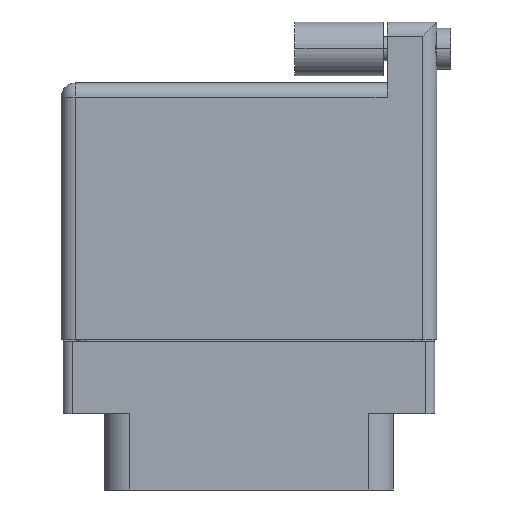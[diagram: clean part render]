
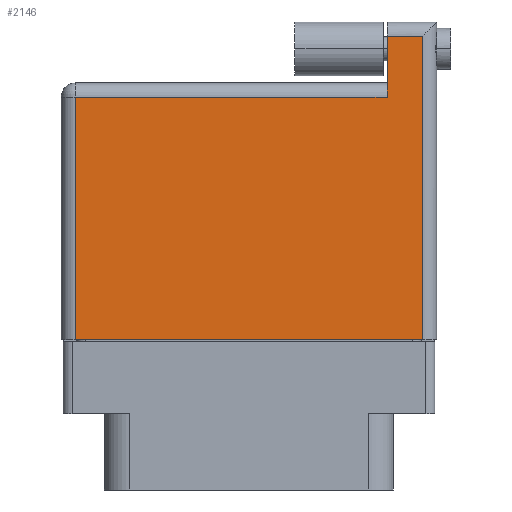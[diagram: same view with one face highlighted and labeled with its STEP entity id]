
A CAD part, front view. The second image highlights one B-rep face of the part: STEP entity #2146.
In plain terms, the highlighted face is planar.
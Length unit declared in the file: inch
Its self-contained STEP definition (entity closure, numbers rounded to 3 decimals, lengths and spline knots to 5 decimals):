
#5 = EDGE_CURVE ( 'NONE', #26352, #6778, #14544, .T. ) ;
#2075 = AXIS2_PLACEMENT_3D ( 'NONE', #9101, #6784, #22873 ) ;
#2146 = ADVANCED_FACE ( 'NONE', ( #16051 ), #13891, .F. ) ;
#3312 = VERTEX_POINT ( 'NONE', #17514 ) ;
#4129 = CARTESIAN_POINT ( 'NONE',  ( -0.6625, 0.97, 0.3575 ) ) ;
#5435 = CARTESIAN_POINT ( 'NONE',  ( 0.4875, 1.02, 0.3575 ) ) ;
#6078 = CARTESIAN_POINT ( 'NONE',  ( -0.6125, -0.1, 0.3575 ) ) ;
#6567 = CARTESIAN_POINT ( 'NONE',  ( 0.4875, 0.97, 0.3575 ) ) ;
#6591 = LINE ( 'NONE', #4129, #15078 ) ;
#6778 = VERTEX_POINT ( 'NONE', #12394 ) ;
#6784 = DIRECTION ( 'NONE',  ( 0., 0., -1. ) ) ;
#7570 = EDGE_CURVE ( 'NONE', #29473, #29462, #14481, .T. ) ;
#8029 = EDGE_CURVE ( 'NONE', #26629, #29473, #13776, .T. ) ;
#8240 = VECTOR ( 'NONE', #25083, 39.37008 ) ;
#9101 = CARTESIAN_POINT ( 'NONE',  ( -0.6625, 0.806, 0.3575 ) ) ;
#9293 = VECTOR ( 'NONE', #26597, 39.37008 ) ;
#10101 = ORIENTED_EDGE ( 'NONE', *, *, #7570, .T. ) ;
#10362 = LINE ( 'NONE', #17004, #9293 ) ;
#11129 = ORIENTED_EDGE ( 'NONE', *, *, #21129, .T. ) ;
#12394 = CARTESIAN_POINT ( 'NONE',  ( 0.4875, 0.756, 0.3575 ) ) ;
#12858 = ORIENTED_EDGE ( 'NONE', *, *, #5, .T. ) ;
#13776 = LINE ( 'NONE', #23210, #20908 ) ;
#13891 = PLANE ( 'NONE',  #2075 ) ;
#14118 = CARTESIAN_POINT ( 'NONE',  ( 0.6125, 0.97, 0.3575 ) ) ;
#14481 = LINE ( 'NONE', #21912, #21490 ) ;
#14544 = LINE ( 'NONE', #5435, #19920 ) ;
#15078 = VECTOR ( 'NONE', #25457, 39.37008 ) ;
#16051 = FACE_OUTER_BOUND ( 'NONE', #21261, .T. ) ;
#16455 = ORIENTED_EDGE ( 'NONE', *, *, #8029, .T. ) ;
#16951 = DIRECTION ( 'NONE',  ( 0., 1., 0. ) ) ;
#17004 = CARTESIAN_POINT ( 'NONE',  ( -0.6125, -0.1, 0.3575 ) ) ;
#17514 = CARTESIAN_POINT ( 'NONE',  ( -0.6125, 0.756, 0.3575 ) ) ;
#18297 = EDGE_CURVE ( 'NONE', #6778, #3312, #20752, .T. ) ;
#18474 = CARTESIAN_POINT ( 'NONE',  ( 0.6125, -0.1, 0.3575 ) ) ;
#19920 = VECTOR ( 'NONE', #24149, 39.37008 ) ;
#20752 = LINE ( 'NONE', #30149, #8240 ) ;
#20908 = VECTOR ( 'NONE', #29831, 39.37008 ) ;
#21129 = EDGE_CURVE ( 'NONE', #29462, #26352, #6591, .T. ) ;
#21261 = EDGE_LOOP ( 'NONE', ( #16455, #10101, #11129, #12858, #28066, #23270 ) ) ;
#21490 = VECTOR ( 'NONE', #16951, 39.37008 ) ;
#21912 = CARTESIAN_POINT ( 'NONE',  ( 0.6125, 1.02, 0.3575 ) ) ;
#22873 = DIRECTION ( 'NONE',  ( -1., 0., 0. ) ) ;
#23210 = CARTESIAN_POINT ( 'NONE',  ( -0.6625, -0.1, 0.3575 ) ) ;
#23270 = ORIENTED_EDGE ( 'NONE', *, *, #28277, .T. ) ;
#24149 = DIRECTION ( 'NONE',  ( 0., -1., 0. ) ) ;
#25083 = DIRECTION ( 'NONE',  ( -1., 0., 0. ) ) ;
#25457 = DIRECTION ( 'NONE',  ( -1., 0., 0. ) ) ;
#26352 = VERTEX_POINT ( 'NONE', #6567 ) ;
#26597 = DIRECTION ( 'NONE',  ( 0., -1., 0. ) ) ;
#26629 = VERTEX_POINT ( 'NONE', #6078 ) ;
#28066 = ORIENTED_EDGE ( 'NONE', *, *, #18297, .T. ) ;
#28277 = EDGE_CURVE ( 'NONE', #3312, #26629, #10362, .T. ) ;
#29462 = VERTEX_POINT ( 'NONE', #14118 ) ;
#29473 = VERTEX_POINT ( 'NONE', #18474 ) ;
#29831 = DIRECTION ( 'NONE',  ( 1., 0., 0. ) ) ;
#30149 = CARTESIAN_POINT ( 'NONE',  ( -0.6625, 0.756, 0.3575 ) ) ;
